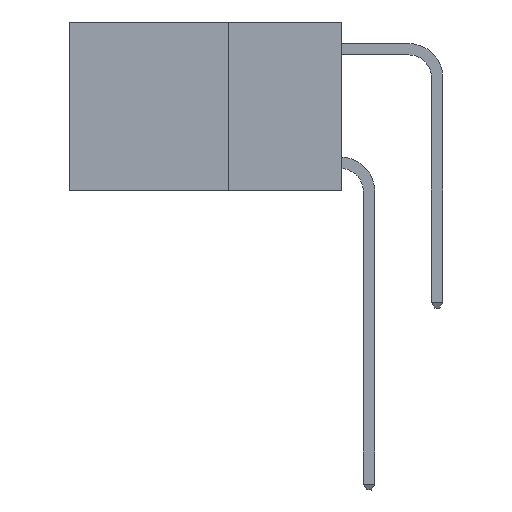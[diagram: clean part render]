
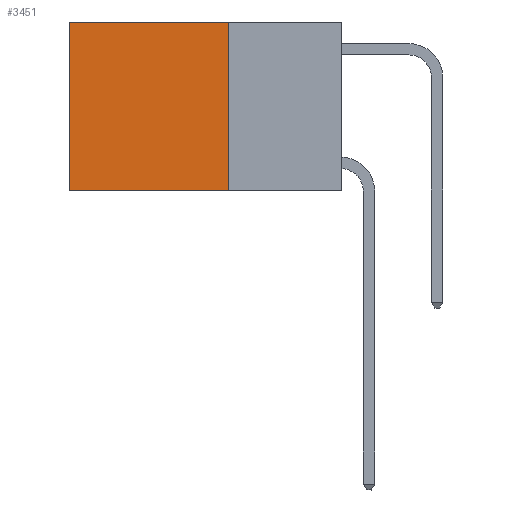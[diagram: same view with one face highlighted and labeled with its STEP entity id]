
A CAD part, left-side view. The second image highlights one B-rep face of the part: STEP entity #3451.
In plain terms, the highlighted planar face has unit normal (-1, 0, 0).
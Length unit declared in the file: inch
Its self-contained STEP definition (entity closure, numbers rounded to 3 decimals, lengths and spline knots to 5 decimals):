
#1257 = DIRECTION ( 'NONE',  ( 0., 0., -1. ) ) ;
#1374 = CARTESIAN_POINT ( 'NONE',  ( 0.2625, 0.25, -0.37 ) ) ;
#2580 = DIRECTION ( 'NONE',  ( 0., 0., -1. ) ) ;
#2811 = LINE ( 'NONE', #12849, #14028 ) ;
#2903 = VERTEX_POINT ( 'NONE', #13156 ) ;
#3451 = ADVANCED_FACE ( 'NONE', ( #10202 ), #5691, .F. ) ;
#3516 = LINE ( 'NONE', #3782, #18588 ) ;
#3782 = CARTESIAN_POINT ( 'NONE',  ( 0.2625, 0.25, -0.37 ) ) ;
#4194 = EDGE_CURVE ( 'NONE', #2903, #10388, #16288, .T. ) ;
#5128 = AXIS2_PLACEMENT_3D ( 'NONE', #18803, #10102, #1257 ) ;
#5448 = LINE ( 'NONE', #9765, #16600 ) ;
#5479 = EDGE_LOOP ( 'NONE', ( #7803, #15427, #6029, #18098 ) ) ;
#5691 = PLANE ( 'NONE',  #5128 ) ;
#6029 = ORIENTED_EDGE ( 'NONE', *, *, #10941, .F. ) ;
#6108 = VERTEX_POINT ( 'NONE', #1374 ) ;
#7217 = VERTEX_POINT ( 'NONE', #18630 ) ;
#7803 = ORIENTED_EDGE ( 'NONE', *, *, #8873, .T. ) ;
#8229 = DIRECTION ( 'NONE',  ( 0., 1., 0. ) ) ;
#8592 = VECTOR ( 'NONE', #14690, 39.37008 ) ;
#8873 = EDGE_CURVE ( 'NONE', #10388, #7217, #2811, .T. ) ;
#9765 = CARTESIAN_POINT ( 'NONE',  ( 0.2625, 0.25, 0. ) ) ;
#10102 = DIRECTION ( 'NONE',  ( 1., 0., 0. ) ) ;
#10202 = FACE_OUTER_BOUND ( 'NONE', #5479, .T. ) ;
#10388 = VERTEX_POINT ( 'NONE', #10606 ) ;
#10606 = CARTESIAN_POINT ( 'NONE',  ( 0.2625, 0.6, 0. ) ) ;
#10941 = EDGE_CURVE ( 'NONE', #2903, #6108, #5448, .T. ) ;
#11245 = DIRECTION ( 'NONE',  ( 0., 0., -1. ) ) ;
#12813 = EDGE_CURVE ( 'NONE', #6108, #7217, #3516, .T. ) ;
#12849 = CARTESIAN_POINT ( 'NONE',  ( 0.2625, 0.6, 0. ) ) ;
#13156 = CARTESIAN_POINT ( 'NONE',  ( 0.2625, 0.25, 0. ) ) ;
#13238 = CARTESIAN_POINT ( 'NONE',  ( 0.2625, 0.25, 0. ) ) ;
#14028 = VECTOR ( 'NONE', #2580, 39.37008 ) ;
#14690 = DIRECTION ( 'NONE',  ( 0., 1., 0. ) ) ;
#15427 = ORIENTED_EDGE ( 'NONE', *, *, #12813, .F. ) ;
#16288 = LINE ( 'NONE', #13238, #8592 ) ;
#16600 = VECTOR ( 'NONE', #11245, 39.37008 ) ;
#18098 = ORIENTED_EDGE ( 'NONE', *, *, #4194, .T. ) ;
#18588 = VECTOR ( 'NONE', #8229, 39.37008 ) ;
#18630 = CARTESIAN_POINT ( 'NONE',  ( 0.2625, 0.6, -0.37 ) ) ;
#18803 = CARTESIAN_POINT ( 'NONE',  ( 0.2625, 0.25, 0. ) ) ;
